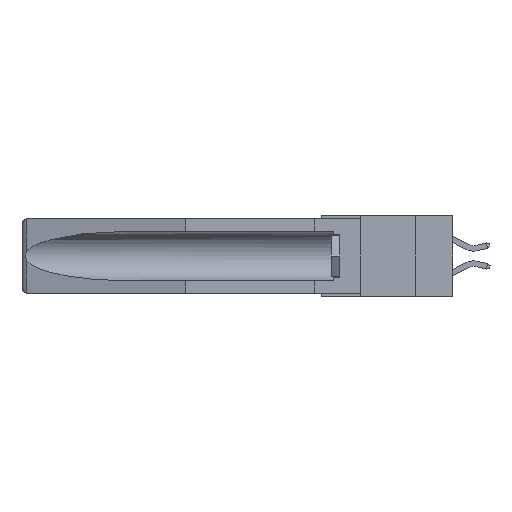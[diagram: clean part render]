
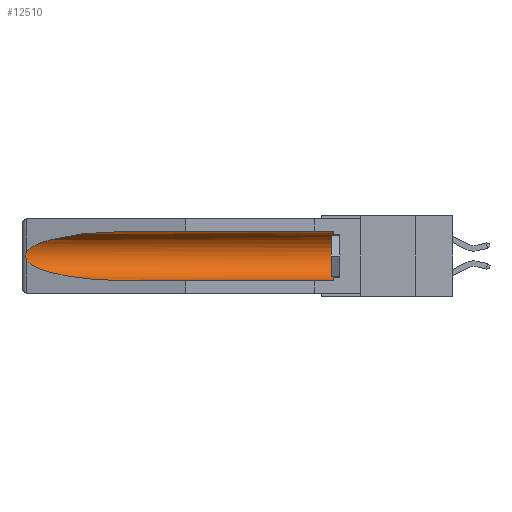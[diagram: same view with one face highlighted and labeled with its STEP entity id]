
A CAD part, left-side view. The second image highlights one B-rep face of the part: STEP entity #12510.
In plain terms, the highlighted cylindrical face has radius 2.857 mm (diameter 5.715 mm), a partial arc.
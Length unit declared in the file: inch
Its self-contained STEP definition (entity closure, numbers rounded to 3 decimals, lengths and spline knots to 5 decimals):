
#238 = CARTESIAN_POINT ( 'NONE',  ( 0.26537, 1.52718, -0.19328 ) ) ;
#271 = ORIENTED_EDGE ( 'NONE', *, *, #1910, .T. ) ;
#351 = CARTESIAN_POINT ( 'NONE',  ( 0.21114, 1.30732, -0.284 ) ) ;
#696 = DIRECTION ( 'NONE',  ( 0., 1., 0. ) ) ;
#1249 = ORIENTED_EDGE ( 'NONE', *, *, #5297, .T. ) ;
#1523 = ORIENTED_EDGE ( 'NONE', *, *, #10912, .T. ) ;
#1555 =( BOUNDED_CURVE ( )  B_SPLINE_CURVE ( 3, ( #16533, #18297, #7972, #9647 ),
 .UNSPECIFIED., .F., .F. ) 
 B_SPLINE_CURVE_WITH_KNOTS ( ( 4, 4 ),
 ( 4.71239, 6.08839 ),
 .UNSPECIFIED. ) 
 CURVE ( )  GEOMETRIC_REPRESENTATION_ITEM ( )  RATIONAL_B_SPLINE_CURVE ( ( 1., 0.848, 0.848, 1. ) ) 
 REPRESENTATION_ITEM ( '' )  );
#1572 = ORIENTED_EDGE ( 'NONE', *, *, #7928, .T. ) ;
#1910 = EDGE_CURVE ( 'NONE', #5828, #7241, #10590, .T. ) ;
#2437 = ORIENTED_EDGE ( 'NONE', *, *, #21454, .T. ) ;
#3268 = CARTESIAN_POINT ( 'NONE',  ( 0.2673, 1.53269, -0.17917 ) ) ;
#3630 =( BOUNDED_CURVE ( )  B_SPLINE_CURVE ( 3, ( #12563, #10735, #351, #17720 ),
 .UNSPECIFIED., .F., .F. ) 
 B_SPLINE_CURVE_WITH_KNOTS ( ( 4, 4 ),
 ( 0.1948, 1.5708 ),
 .UNSPECIFIED. ) 
 CURVE ( )  GEOMETRIC_REPRESENTATION_ITEM ( )  RATIONAL_B_SPLINE_CURVE ( ( 1., 0.848, 0.848, 1. ) ) 
 REPRESENTATION_ITEM ( '' )  );
#4091 = VECTOR ( 'NONE', #696, 39.37008 ) ;
#4102 = DIRECTION ( 'NONE',  ( 0., 1., 0. ) ) ;
#4556 = CARTESIAN_POINT ( 'NONE',  ( 0.155, 1.07973, -0.059 ) ) ;
#4606 = AXIS2_PLACEMENT_3D ( 'NONE', #22243, #6639, #8516 ) ;
#5297 = EDGE_CURVE ( 'NONE', #7241, #21135, #14832, .T. ) ;
#5828 = VERTEX_POINT ( 'NONE', #21536 ) ;
#6639 = DIRECTION ( 'NONE',  ( 0., -1., 0. ) ) ;
#6692 = CARTESIAN_POINT ( 'NONE',  ( 0.26654, 1.53092, -0.15636 ) ) ;
#6758 = CARTESIAN_POINT ( 'NONE',  ( 0.2675, 1.53308, -0.17534 ) ) ;
#7077 = CARTESIAN_POINT ( 'NONE',  ( 0.155, 0.126, -0.059 ) ) ;
#7241 = VERTEX_POINT ( 'NONE', #7077 ) ;
#7928 = EDGE_CURVE ( 'NONE', #21135, #15434, #1555, .T. ) ;
#7972 = CARTESIAN_POINT ( 'NONE',  ( 0.25451, 1.48313, -0.09465 ) ) ;
#8360 = FACE_OUTER_BOUND ( 'NONE', #16186, .T. ) ;
#8494 = CARTESIAN_POINT ( 'NONE',  ( 0.26537, 1.52718, -0.19328 ) ) ;
#8516 = DIRECTION ( 'NONE',  ( 0., 0., 1. ) ) ;
#8568 = CARTESIAN_POINT ( 'NONE',  ( 0.2673, 1.5327, -0.16383 ) ) ;
#9647 = CARTESIAN_POINT ( 'NONE',  ( 0.26537, 1.52718, -0.14972 ) ) ;
#10582 = LINE ( 'NONE', #14272, #4091 ) ;
#10590 = CIRCLE ( 'NONE', #4606, 0.1125 ) ;
#10735 = CARTESIAN_POINT ( 'NONE',  ( 0.25451, 1.48313, -0.24835 ) ) ;
#10912 = EDGE_CURVE ( 'NONE', #13656, #14029, #3630, .T. ) ;
#11928 = CARTESIAN_POINT ( 'NONE',  ( 0.26537, 1.52718, -0.14972 ) ) ;
#12510 = ADVANCED_FACE ( 'NONE', ( #8360 ), #16503, .F. ) ;
#12563 = CARTESIAN_POINT ( 'NONE',  ( 0.26537, 1.52718, -0.19328 ) ) ;
#12737 = CARTESIAN_POINT ( 'NONE',  ( 0.26537, 1.52718, -0.14972 ) ) ;
#13258 = CARTESIAN_POINT ( 'NONE',  ( 0.155, 1.07973, -0.284 ) ) ;
#13655 = CARTESIAN_POINT ( 'NONE',  ( 0.2675, 1.53308, -0.16763 ) ) ;
#13656 = VERTEX_POINT ( 'NONE', #238 ) ;
#14029 = VERTEX_POINT ( 'NONE', #13258 ) ;
#14272 = CARTESIAN_POINT ( 'NONE',  ( 0.155, -0.30754, -0.284 ) ) ;
#14491 = CARTESIAN_POINT ( 'NONE',  ( 0.155, -0.30754, -0.1715 ) ) ;
#14832 = LINE ( 'NONE', #20947, #19160 ) ;
#14894 = ORIENTED_EDGE ( 'NONE', *, *, #19224, .F. ) ;
#15434 = VERTEX_POINT ( 'NONE', #12737 ) ;
#16186 = EDGE_LOOP ( 'NONE', ( #1572, #2437, #1523, #14894, #271, #1249 ) ) ;
#16230 = DIRECTION ( 'NONE',  ( 0., 0., 1. ) ) ;
#16503 = CYLINDRICAL_SURFACE ( 'NONE', #17670, 0.1125 ) ;
#16533 = CARTESIAN_POINT ( 'NONE',  ( 0.155, 1.07973, -0.059 ) ) ;
#17132 = CARTESIAN_POINT ( 'NONE',  ( 0.26655, 1.53094, -0.18657 ) ) ;
#17216 = CARTESIAN_POINT ( 'NONE',  ( 0.26597, 1.52961, -0.15275 ) ) ;
#17670 = AXIS2_PLACEMENT_3D ( 'NONE', #14491, #4102, #16230 ) ;
#17720 = CARTESIAN_POINT ( 'NONE',  ( 0.155, 1.07973, -0.284 ) ) ;
#18297 = CARTESIAN_POINT ( 'NONE',  ( 0.21114, 1.30732, -0.059 ) ) ;
#18887 = CARTESIAN_POINT ( 'NONE',  ( 0.26597, 1.5296, -0.19026 ) ) ;
#19160 = VECTOR ( 'NONE', #20874, 39.37008 ) ;
#19224 = EDGE_CURVE ( 'NONE', #5828, #14029, #10582, .T. ) ;
#20874 = DIRECTION ( 'NONE',  ( 0., 1., 0. ) ) ;
#20947 = CARTESIAN_POINT ( 'NONE',  ( 0.155, -0.30754, -0.059 ) ) ;
#21135 = VERTEX_POINT ( 'NONE', #4556 ) ;
#21454 = EDGE_CURVE ( 'NONE', #15434, #13656, #22403, .T. ) ;
#21536 = CARTESIAN_POINT ( 'NONE',  ( 0.155, 0.126, -0.284 ) ) ;
#22243 = CARTESIAN_POINT ( 'NONE',  ( 0.155, 0.126, -0.1715 ) ) ;
#22403 = B_SPLINE_CURVE_WITH_KNOTS ( 'NONE', 3,
 ( #11928, #17216, #6692, #8568, #13655, #6758, #3268, #17132, #18887, #8494 ),
 .UNSPECIFIED., .F., .F.,
 ( 4, 2, 2, 2, 4 ),
 ( 0., 0.00029, 0.00058, 0.00087, 0.00117 ),
 .UNSPECIFIED. ) ;
